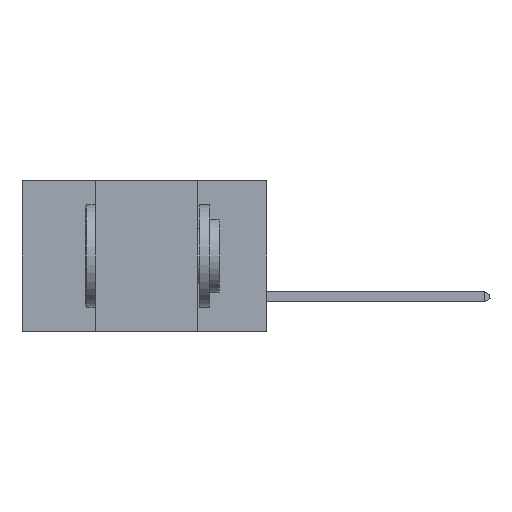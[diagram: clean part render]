
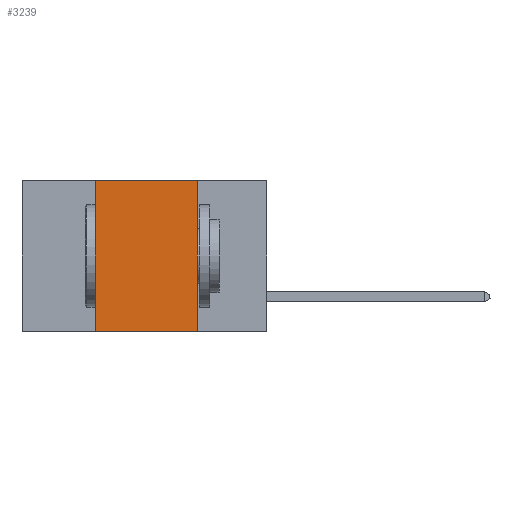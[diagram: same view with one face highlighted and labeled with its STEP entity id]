
A CAD part, left-side view. The second image highlights one B-rep face of the part: STEP entity #3239.
In plain terms, the highlighted planar face has unit normal (-1, 0, 0).
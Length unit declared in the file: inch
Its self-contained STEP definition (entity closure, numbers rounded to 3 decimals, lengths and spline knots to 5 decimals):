
#689 = ORIENTED_EDGE ( 'NONE', *, *, #2347, .F. ) ;
#965 = CARTESIAN_POINT ( 'NONE',  ( 0., 0.42, 0. ) ) ;
#1568 = ORIENTED_EDGE ( 'NONE', *, *, #3334, .F. ) ;
#2226 = FACE_OUTER_BOUND ( 'NONE', #12603, .T. ) ;
#2347 = EDGE_CURVE ( 'NONE', #12241, #13679, #22344, .T. ) ;
#3239 = ADVANCED_FACE ( 'NONE', ( #2226 ), #15976, .F. ) ;
#3334 = EDGE_CURVE ( 'NONE', #13679, #18171, #18922, .T. ) ;
#3953 = LINE ( 'NONE', #10355, #15740 ) ;
#4101 = VECTOR ( 'NONE', #20875, 39.37008 ) ;
#4880 = ORIENTED_EDGE ( 'NONE', *, *, #8282, .F. ) ;
#5212 = CARTESIAN_POINT ( 'NONE',  ( 0., 0.6, 0. ) ) ;
#5955 = CARTESIAN_POINT ( 'NONE',  ( 0., 0.6, 0. ) ) ;
#6100 = AXIS2_PLACEMENT_3D ( 'NONE', #5955, #8115, #7939 ) ;
#7939 = DIRECTION ( 'NONE',  ( 0., 0., -1. ) ) ;
#8115 = DIRECTION ( 'NONE',  ( 1., 0., 0. ) ) ;
#8282 = EDGE_CURVE ( 'NONE', #14189, #12241, #12178, .T. ) ;
#9057 = CARTESIAN_POINT ( 'NONE',  ( 0., 0.17, -0.37 ) ) ;
#10355 = CARTESIAN_POINT ( 'NONE',  ( 0., 0.6, -0.37 ) ) ;
#10633 = CARTESIAN_POINT ( 'NONE',  ( 0., 0.17, 0. ) ) ;
#11015 = EDGE_CURVE ( 'NONE', #14189, #18171, #3953, .T. ) ;
#12178 = LINE ( 'NONE', #15272, #13106 ) ;
#12241 = VERTEX_POINT ( 'NONE', #965 ) ;
#12508 = VECTOR ( 'NONE', #13291, 39.37008 ) ;
#12603 = EDGE_LOOP ( 'NONE', ( #1568, #689, #4880, #17414 ) ) ;
#13106 = VECTOR ( 'NONE', #23280, 39.37008 ) ;
#13291 = DIRECTION ( 'NONE',  ( 0., -1., 0. ) ) ;
#13679 = VERTEX_POINT ( 'NONE', #23842 ) ;
#14189 = VERTEX_POINT ( 'NONE', #20899 ) ;
#15272 = CARTESIAN_POINT ( 'NONE',  ( 0., 0.42, 0. ) ) ;
#15740 = VECTOR ( 'NONE', #21957, 39.37008 ) ;
#15976 = PLANE ( 'NONE',  #6100 ) ;
#17414 = ORIENTED_EDGE ( 'NONE', *, *, #11015, .T. ) ;
#18171 = VERTEX_POINT ( 'NONE', #9057 ) ;
#18922 = LINE ( 'NONE', #10633, #4101 ) ;
#20875 = DIRECTION ( 'NONE',  ( 0., 0., -1. ) ) ;
#20899 = CARTESIAN_POINT ( 'NONE',  ( 0., 0.42, -0.37 ) ) ;
#21957 = DIRECTION ( 'NONE',  ( 0., -1., 0. ) ) ;
#22344 = LINE ( 'NONE', #5212, #12508 ) ;
#23280 = DIRECTION ( 'NONE',  ( 0., 0., 1. ) ) ;
#23842 = CARTESIAN_POINT ( 'NONE',  ( 0., 0.17, 0. ) ) ;
